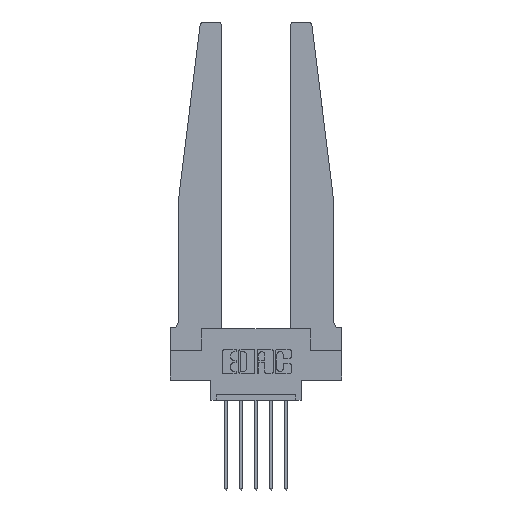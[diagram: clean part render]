
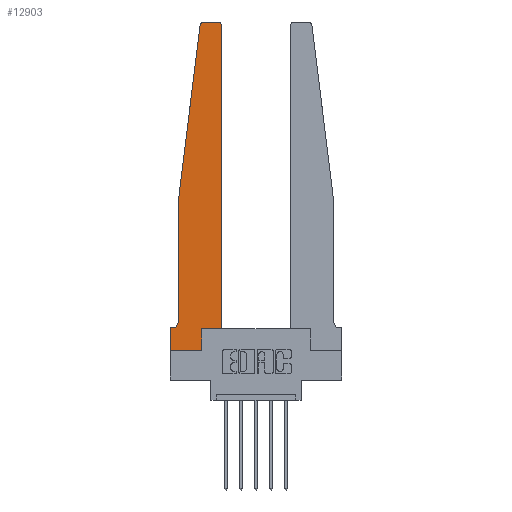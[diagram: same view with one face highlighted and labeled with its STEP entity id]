
A CAD part, top view. The second image highlights one B-rep face of the part: STEP entity #12903.
In plain terms, the highlighted planar face has unit normal (0, 0, 1).
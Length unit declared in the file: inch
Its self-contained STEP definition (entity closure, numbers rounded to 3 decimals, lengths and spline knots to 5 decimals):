
#41 = EDGE_CURVE ( 'NONE', #2380, #6715, #1977, .T. ) ;
#136 = PLANE ( 'NONE',  #895 ) ;
#157 = CARTESIAN_POINT ( 'NONE',  ( 0.2605, 0.18, 0.37 ) ) ;
#350 = DIRECTION ( 'NONE',  ( 1., 0., 0. ) ) ;
#461 = VECTOR ( 'NONE', #11830, 39.37008 ) ;
#770 = CARTESIAN_POINT ( 'NONE',  ( 0.24675, 2.72367, 0.37 ) ) ;
#895 = AXIS2_PLACEMENT_3D ( 'NONE', #9641, #6508, #9502 ) ;
#926 = ORIENTED_EDGE ( 'NONE', *, *, #3080, .T. ) ;
#1018 = CARTESIAN_POINT ( 'NONE',  ( 0., 0., 0.37 ) ) ;
#1042 = ORIENTED_EDGE ( 'NONE', *, *, #2405, .T. ) ;
#1218 = VECTOR ( 'NONE', #5994, 39.37008 ) ;
#1294 = ORIENTED_EDGE ( 'NONE', *, *, #1741, .T. ) ;
#1301 = EDGE_CURVE ( 'NONE', #2283, #9414, #1532, .T. ) ;
#1334 = CARTESIAN_POINT ( 'NONE',  ( 0.2605, 0., 0.37 ) ) ;
#1338 = CIRCLE ( 'NONE', #4142, 0.05 ) ;
#1418 = CARTESIAN_POINT ( 'NONE',  ( 0.27653, 2.75, 0.37 ) ) ;
#1442 = CARTESIAN_POINT ( 'NONE',  ( 0.065, 1.25, 0.37 ) ) ;
#1469 = ORIENTED_EDGE ( 'NONE', *, *, #1557, .T. ) ;
#1532 = CIRCLE ( 'NONE', #13233, 0.03 ) ;
#1557 = EDGE_CURVE ( 'NONE', #11689, #7676, #1338, .T. ) ;
#1654 = CARTESIAN_POINT ( 'NONE',  ( 0.015, 0.1875, 0.37 ) ) ;
#1741 = EDGE_CURVE ( 'NONE', #9264, #6443, #7135, .T. ) ;
#1977 = LINE ( 'NONE', #12184, #1218 ) ;
#2123 = EDGE_CURVE ( 'NONE', #7676, #5213, #7546, .T. ) ;
#2166 = VECTOR ( 'NONE', #8281, 39.37008 ) ;
#2281 = ORIENTED_EDGE ( 'NONE', *, *, #10853, .T. ) ;
#2283 = VERTEX_POINT ( 'NONE', #8979 ) ;
#2380 = VERTEX_POINT ( 'NONE', #1334 ) ;
#2405 = EDGE_CURVE ( 'NONE', #6715, #9196, #5496, .T. ) ;
#2413 = DIRECTION ( 'NONE',  ( -1., 0., 0. ) ) ;
#2507 = CARTESIAN_POINT ( 'NONE',  ( 0.425, 0.18, 0.37 ) ) ;
#2591 = ORIENTED_EDGE ( 'NONE', *, *, #6154, .T. ) ;
#2758 = ORIENTED_EDGE ( 'NONE', *, *, #6647, .T. ) ;
#3054 = AXIS2_PLACEMENT_3D ( 'NONE', #4361, #8494, #7475 ) ;
#3080 = EDGE_CURVE ( 'NONE', #6443, #11689, #5537, .T. ) ;
#3632 = LINE ( 'NONE', #11931, #11739 ) ;
#4142 = AXIS2_PLACEMENT_3D ( 'NONE', #9941, #5802, #2413 ) ;
#4240 = CARTESIAN_POINT ( 'NONE',  ( 0.065, 1.25, 0.37 ) ) ;
#4361 = CARTESIAN_POINT ( 'NONE',  ( 0.27653, 2.72, 0.37 ) ) ;
#4386 = LINE ( 'NONE', #8513, #11174 ) ;
#4731 = CARTESIAN_POINT ( 'NONE',  ( 0.065, 0.2375, 0.37 ) ) ;
#4735 = DIRECTION ( 'NONE',  ( 1., 0., 0. ) ) ;
#5213 = VERTEX_POINT ( 'NONE', #11307 ) ;
#5496 = LINE ( 'NONE', #6527, #11572 ) ;
#5537 = LINE ( 'NONE', #1442, #10710 ) ;
#5672 = LINE ( 'NONE', #2507, #12490 ) ;
#5802 = DIRECTION ( 'NONE',  ( 0., 0., -1. ) ) ;
#5994 = DIRECTION ( 'NONE',  ( 0., 1., 0. ) ) ;
#6025 = LINE ( 'NONE', #7962, #461 ) ;
#6140 = DIRECTION ( 'NONE',  ( 1., 0., 0. ) ) ;
#6154 = EDGE_CURVE ( 'NONE', #5213, #11093, #4386, .T. ) ;
#6443 = VERTEX_POINT ( 'NONE', #10926 ) ;
#6508 = DIRECTION ( 'NONE',  ( 0., 0., 1. ) ) ;
#6527 = CARTESIAN_POINT ( 'NONE',  ( 0.425, 0.18, 0.37 ) ) ;
#6647 = EDGE_CURVE ( 'NONE', #9196, #2283, #5672, .T. ) ;
#6715 = VERTEX_POINT ( 'NONE', #157 ) ;
#6881 = ORIENTED_EDGE ( 'NONE', *, *, #12648, .T. ) ;
#7074 = CARTESIAN_POINT ( 'NONE',  ( 0.395, 2.72, 0.37 ) ) ;
#7135 = LINE ( 'NONE', #4240, #2166 ) ;
#7138 = DIRECTION ( 'NONE',  ( 0., 0., 1. ) ) ;
#7475 = DIRECTION ( 'NONE',  ( 1., 0., 0. ) ) ;
#7524 = FACE_OUTER_BOUND ( 'NONE', #7948, .T. ) ;
#7546 = LINE ( 'NONE', #11866, #12196 ) ;
#7676 = VERTEX_POINT ( 'NONE', #1654 ) ;
#7948 = EDGE_LOOP ( 'NONE', ( #13199, #6881, #1294, #926, #1469, #11880, #2591, #2281, #11556, #1042, #2758, #13138 ) ) ;
#7962 = CARTESIAN_POINT ( 'NONE',  ( 0.25, 2.75, 0.37 ) ) ;
#8281 = DIRECTION ( 'NONE',  ( -0.122, -0.992, 0. ) ) ;
#8494 = DIRECTION ( 'NONE',  ( 0., 0., 1. ) ) ;
#8495 = CARTESIAN_POINT ( 'NONE',  ( 0.425, 0.18, 0.37 ) ) ;
#8513 = CARTESIAN_POINT ( 'NONE',  ( 0., 0., 0.37 ) ) ;
#8570 = DIRECTION ( 'NONE',  ( -1., 0., 0. ) ) ;
#8803 = DIRECTION ( 'NONE',  ( 0., -1., 0. ) ) ;
#8979 = CARTESIAN_POINT ( 'NONE',  ( 0.425, 2.72, 0.37 ) ) ;
#9196 = VERTEX_POINT ( 'NONE', #8495 ) ;
#9264 = VERTEX_POINT ( 'NONE', #770 ) ;
#9414 = VERTEX_POINT ( 'NONE', #11306 ) ;
#9502 = DIRECTION ( 'NONE',  ( 1., 0., 0. ) ) ;
#9641 = CARTESIAN_POINT ( 'NONE',  ( 0., 0.1875, 0.37 ) ) ;
#9752 = DIRECTION ( 'NONE',  ( 0., 1., 0. ) ) ;
#9941 = CARTESIAN_POINT ( 'NONE',  ( 0.015, 0.2375, 0.37 ) ) ;
#10174 = DIRECTION ( 'NONE',  ( 0., -1., 0. ) ) ;
#10710 = VECTOR ( 'NONE', #8803, 39.37008 ) ;
#10811 = VERTEX_POINT ( 'NONE', #1418 ) ;
#10853 = EDGE_CURVE ( 'NONE', #11093, #2380, #3632, .T. ) ;
#10926 = CARTESIAN_POINT ( 'NONE',  ( 0.065, 1.25, 0.37 ) ) ;
#11093 = VERTEX_POINT ( 'NONE', #1018 ) ;
#11174 = VECTOR ( 'NONE', #10174, 39.37008 ) ;
#11306 = CARTESIAN_POINT ( 'NONE',  ( 0.395, 2.75, 0.37 ) ) ;
#11307 = CARTESIAN_POINT ( 'NONE',  ( 0., 0.1875, 0.37 ) ) ;
#11556 = ORIENTED_EDGE ( 'NONE', *, *, #41, .T. ) ;
#11572 = VECTOR ( 'NONE', #350, 39.37008 ) ;
#11689 = VERTEX_POINT ( 'NONE', #4731 ) ;
#11739 = VECTOR ( 'NONE', #4735, 39.37008 ) ;
#11830 = DIRECTION ( 'NONE',  ( -1., 0., 0. ) ) ;
#11866 = CARTESIAN_POINT ( 'NONE',  ( 0.065, 0.1875, 0.37 ) ) ;
#11880 = ORIENTED_EDGE ( 'NONE', *, *, #2123, .T. ) ;
#11931 = CARTESIAN_POINT ( 'NONE',  ( 0., 0., 0.37 ) ) ;
#12184 = CARTESIAN_POINT ( 'NONE',  ( 0.2605, 0.18, 0.37 ) ) ;
#12196 = VECTOR ( 'NONE', #8570, 39.37008 ) ;
#12274 = EDGE_CURVE ( 'NONE', #9414, #10811, #6025, .T. ) ;
#12490 = VECTOR ( 'NONE', #9752, 39.37008 ) ;
#12648 = EDGE_CURVE ( 'NONE', #10811, #9264, #13245, .T. ) ;
#12903 = ADVANCED_FACE ( 'NONE', ( #7524 ), #136, .T. ) ;
#13138 = ORIENTED_EDGE ( 'NONE', *, *, #1301, .T. ) ;
#13199 = ORIENTED_EDGE ( 'NONE', *, *, #12274, .T. ) ;
#13233 = AXIS2_PLACEMENT_3D ( 'NONE', #7074, #7138, #6140 ) ;
#13245 = CIRCLE ( 'NONE', #3054, 0.03 ) ;
